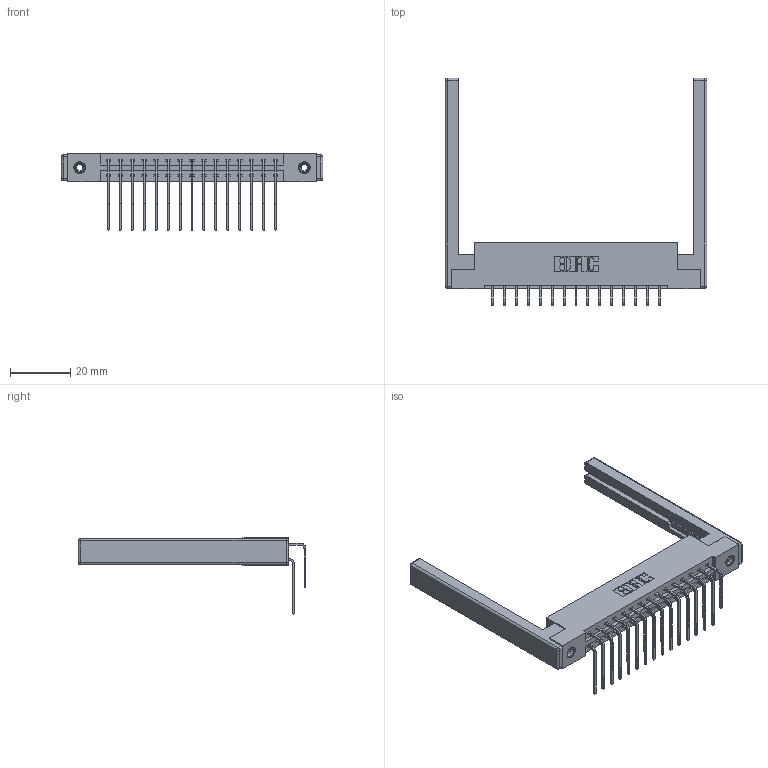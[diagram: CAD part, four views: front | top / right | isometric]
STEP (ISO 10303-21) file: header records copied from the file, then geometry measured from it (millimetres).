
FILE_DESCRIPTION (( 'STEP AP203' ), '1' );
FILE_NAME ('387-030-559-268.STEP', '2019-10-17T15:09:06', ( '' ), ( '' ), 'SwSTEP 2.0', 'SolidWorks 2016', '' );
FILE_SCHEMA (( 'CONFIG_CONTROL_DESIGN' ));
Length unit declared in the file: inch
Products named in the file (6): 387-030-559-268; 345-250-001_345-250-001-102; 337 Part_Flush Mounting Lugs - 0.156 Dia-TI; 307-220-068; 345-292-001_559 Tail - 2; 345-292-001_558 559 Tail - 1
Assembly tree (35 placements, depth 2):
  387-030-559-268
    337 Part_Flush Mounting Lugs - 0.156 Dia-TI
    345-292-001_558 559 Tail - 1  x15
    345-292-001_559 Tail - 2  x15
    345-250-001_345-250-001-102  x2
    307-220-068  x2
Bounding box: 86.87 x 75.63 x 25.53 mm (x, y, z)
Volume: 13353.3 mm3; surface area: 14780 mm2
Topology: 35 solids, 35 shells, 1948 faces, 5711 edges, 3746 vertices
Faces by surface type: plane 1358, cylinder 566, cone 12, sphere 8, torus 4
Entity records: 19666 total; most frequent: CARTESIAN_POINT 3346, ORIENTED_EDGE 3220, DIRECTION 2948, EDGE_CURVE 1610, VECTOR 1392, LINE 1392, VERTEX_POINT 1062, AXIS2_PLACEMENT_3D 778
